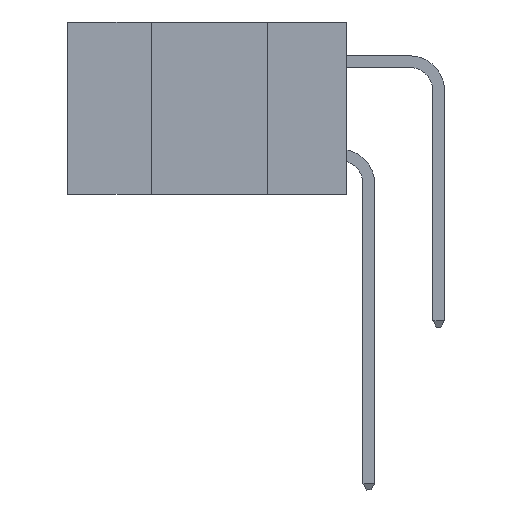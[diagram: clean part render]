
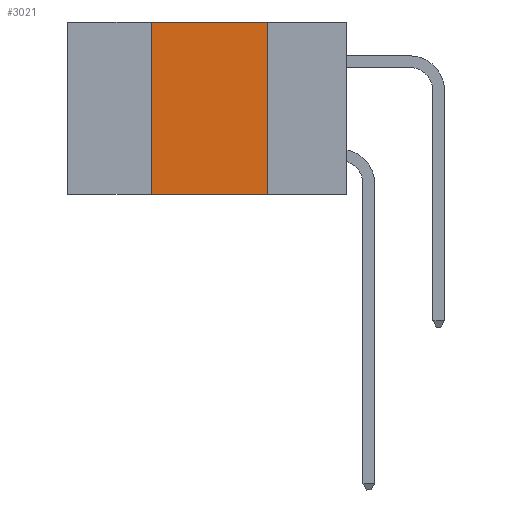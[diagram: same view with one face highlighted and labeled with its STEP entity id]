
A CAD part, left-side view. The second image highlights one B-rep face of the part: STEP entity #3021.
In plain terms, the highlighted planar face has unit normal (-1, 0, 0).
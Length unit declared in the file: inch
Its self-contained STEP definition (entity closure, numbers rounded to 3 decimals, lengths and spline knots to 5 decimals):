
#465 = VECTOR ( 'NONE', #1205, 39.37008 ) ;
#1205 = DIRECTION ( 'NONE',  ( 0., 0., 1. ) ) ;
#1655 = VERTEX_POINT ( 'NONE', #7208 ) ;
#2060 = PLANE ( 'NONE',  #7206 ) ;
#3021 = ADVANCED_FACE ( 'NONE', ( #15625 ), #2060, .F. ) ;
#4223 = DIRECTION ( 'NONE',  ( 0., 0., -1. ) ) ;
#4610 = DIRECTION ( 'NONE',  ( 1., 0., 0. ) ) ;
#5237 = EDGE_CURVE ( 'NONE', #12553, #1655, #14131, .T. ) ;
#5487 = VERTEX_POINT ( 'NONE', #12893 ) ;
#6547 = EDGE_CURVE ( 'NONE', #13432, #12553, #10736, .T. ) ;
#7206 = AXIS2_PLACEMENT_3D ( 'NONE', #8005, #4610, #4223 ) ;
#7208 = CARTESIAN_POINT ( 'NONE',  ( 0., 0.17, -0.37 ) ) ;
#7372 = EDGE_CURVE ( 'NONE', #5487, #1655, #14063, .T. ) ;
#7379 = LINE ( 'NONE', #8889, #465 ) ;
#8005 = CARTESIAN_POINT ( 'NONE',  ( 0., 0.6, 0. ) ) ;
#8127 = DIRECTION ( 'NONE',  ( 0., 0., -1. ) ) ;
#8446 = CARTESIAN_POINT ( 'NONE',  ( 0., 0.17, 0. ) ) ;
#8757 = ORIENTED_EDGE ( 'NONE', *, *, #12820, .F. ) ;
#8889 = CARTESIAN_POINT ( 'NONE',  ( 0., 0.42, 0. ) ) ;
#9145 = ORIENTED_EDGE ( 'NONE', *, *, #7372, .T. ) ;
#10123 = CARTESIAN_POINT ( 'NONE',  ( 0., 0.42, 0. ) ) ;
#10347 = VECTOR ( 'NONE', #14693, 39.37008 ) ;
#10661 = ORIENTED_EDGE ( 'NONE', *, *, #5237, .F. ) ;
#10710 = VECTOR ( 'NONE', #16236, 39.37008 ) ;
#10736 = LINE ( 'NONE', #14640, #10347 ) ;
#11533 = EDGE_LOOP ( 'NONE', ( #10661, #11880, #8757, #9145 ) ) ;
#11880 = ORIENTED_EDGE ( 'NONE', *, *, #6547, .F. ) ;
#12078 = CARTESIAN_POINT ( 'NONE',  ( 0., 0.17, 0. ) ) ;
#12553 = VERTEX_POINT ( 'NONE', #12078 ) ;
#12820 = EDGE_CURVE ( 'NONE', #5487, #13432, #7379, .T. ) ;
#12893 = CARTESIAN_POINT ( 'NONE',  ( 0., 0.42, -0.37 ) ) ;
#13432 = VERTEX_POINT ( 'NONE', #10123 ) ;
#13783 = CARTESIAN_POINT ( 'NONE',  ( 0., 0.6, -0.37 ) ) ;
#14063 = LINE ( 'NONE', #13783, #10710 ) ;
#14131 = LINE ( 'NONE', #8446, #14517 ) ;
#14517 = VECTOR ( 'NONE', #8127, 39.37008 ) ;
#14640 = CARTESIAN_POINT ( 'NONE',  ( 0., 0.6, 0. ) ) ;
#14693 = DIRECTION ( 'NONE',  ( 0., -1., 0. ) ) ;
#15625 = FACE_OUTER_BOUND ( 'NONE', #11533, .T. ) ;
#16236 = DIRECTION ( 'NONE',  ( 0., -1., 0. ) ) ;
